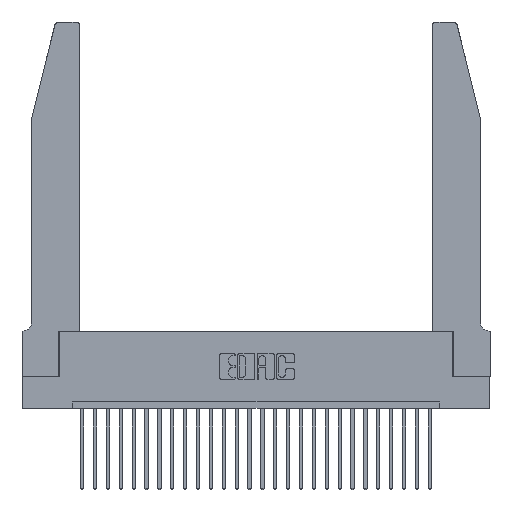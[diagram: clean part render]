
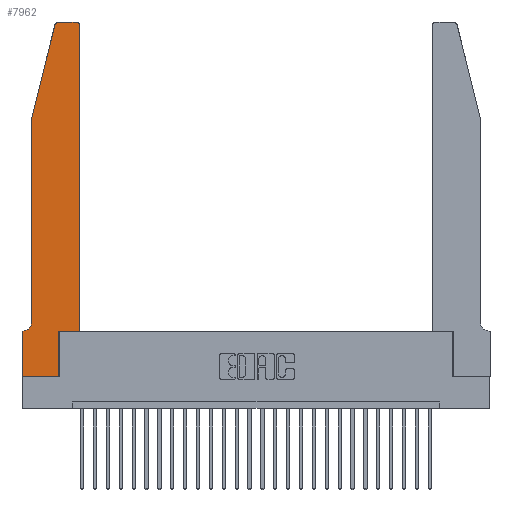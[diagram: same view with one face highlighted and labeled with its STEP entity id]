
A CAD part, top view. The second image highlights one B-rep face of the part: STEP entity #7962.
In plain terms, the highlighted planar face has unit normal (0, 0, 1).
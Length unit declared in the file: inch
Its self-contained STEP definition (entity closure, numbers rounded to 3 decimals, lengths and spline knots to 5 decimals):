
#23 = CARTESIAN_POINT ( 'NONE',  ( 0.0055, 0.42, 0.37 ) ) ;
#168 = CARTESIAN_POINT ( 'NONE',  ( 0.2865, 0.35, 0.37 ) ) ;
#391 = EDGE_CURVE ( 'NONE', #25105, #6199, #17100, .T. ) ;
#398 = FACE_OUTER_BOUND ( 'NONE', #26909, .T. ) ;
#477 = VERTEX_POINT ( 'NONE', #11469 ) ;
#653 = CARTESIAN_POINT ( 'NONE',  ( 0.4205, 2.72, 0.37 ) ) ;
#956 = CIRCLE ( 'NONE', #12991, 0.03 ) ;
#1364 = EDGE_CURVE ( 'NONE', #17092, #24088, #25146, .T. ) ;
#1697 = VECTOR ( 'NONE', #10542, 39.37008 ) ;
#2000 = ORIENTED_EDGE ( 'NONE', *, *, #7348, .T. ) ;
#2100 = EDGE_CURVE ( 'NONE', #6119, #6591, #956, .T. ) ;
#2152 = VERTEX_POINT ( 'NONE', #21927 ) ;
#2568 = DIRECTION ( 'NONE',  ( 0., 0., 1. ) ) ;
#2609 = VECTOR ( 'NONE', #7868, 39.37008 ) ;
#2781 = CARTESIAN_POINT ( 'NONE',  ( 0.0055, 0.35, 0.37 ) ) ;
#4264 = AXIS2_PLACEMENT_3D ( 'NONE', #653, #2568, #6872 ) ;
#4354 = CARTESIAN_POINT ( 'NONE',  ( 0.25487, 2.72718, 0.37 ) ) ;
#4357 = DIRECTION ( 'NONE',  ( 0., 0., -1. ) ) ;
#5154 = DIRECTION ( 'NONE',  ( 0., 0., 1. ) ) ;
#5604 = EDGE_CURVE ( 'NONE', #6199, #19253, #10950, .T. ) ;
#5846 = ORIENTED_EDGE ( 'NONE', *, *, #10791, .T. ) ;
#5909 = VECTOR ( 'NONE', #23273, 39.37008 ) ;
#6119 = VERTEX_POINT ( 'NONE', #7009 ) ;
#6199 = VERTEX_POINT ( 'NONE', #15325 ) ;
#6318 = CARTESIAN_POINT ( 'NONE',  ( 0.0755, 0.35, 0.37 ) ) ;
#6411 = ORIENTED_EDGE ( 'NONE', *, *, #20065, .T. ) ;
#6591 = VERTEX_POINT ( 'NONE', #4354 ) ;
#6872 = DIRECTION ( 'NONE',  ( 1., 0., 0. ) ) ;
#6919 = EDGE_CURVE ( 'NONE', #12487, #25379, #16884, .T. ) ;
#6983 = DIRECTION ( 'NONE',  ( 1., 0., 0. ) ) ;
#7009 = CARTESIAN_POINT ( 'NONE',  ( 0.284, 2.75, 0.37 ) ) ;
#7058 = CARTESIAN_POINT ( 'NONE',  ( 0.284, 2.72, 0.37 ) ) ;
#7182 = DIRECTION ( 'NONE',  ( 1., 0., 0. ) ) ;
#7336 = CARTESIAN_POINT ( 'NONE',  ( 0.0755, 0.42, 0.37 ) ) ;
#7348 = EDGE_CURVE ( 'NONE', #25379, #17092, #19208, .T. ) ;
#7567 = ORIENTED_EDGE ( 'NONE', *, *, #13191, .T. ) ;
#7577 = ORIENTED_EDGE ( 'NONE', *, *, #1364, .T. ) ;
#7868 = DIRECTION ( 'NONE',  ( -0.239, -0.971, 0. ) ) ;
#7962 = ADVANCED_FACE ( 'NONE', ( #398 ), #11408, .T. ) ;
#8135 = ORIENTED_EDGE ( 'NONE', *, *, #6919, .T. ) ;
#8863 = VECTOR ( 'NONE', #11765, 39.37008 ) ;
#10542 = DIRECTION ( 'NONE',  ( -1., 0., 0. ) ) ;
#10791 = EDGE_CURVE ( 'NONE', #6591, #12487, #27391, .T. ) ;
#10950 = LINE ( 'NONE', #14642, #5909 ) ;
#11408 = PLANE ( 'NONE',  #21002 ) ;
#11469 = CARTESIAN_POINT ( 'NONE',  ( 0.4505, 2.72, 0.37 ) ) ;
#11477 = DIRECTION ( 'NONE',  ( 0., 0., 1. ) ) ;
#11765 = DIRECTION ( 'NONE',  ( 0., -1., 0. ) ) ;
#12487 = VERTEX_POINT ( 'NONE', #23101 ) ;
#12876 = EDGE_CURVE ( 'NONE', #2152, #25105, #24219, .T. ) ;
#12991 = AXIS2_PLACEMENT_3D ( 'NONE', #7058, #11477, #6983 ) ;
#13191 = EDGE_CURVE ( 'NONE', #24088, #2152, #14501, .T. ) ;
#13515 = CARTESIAN_POINT ( 'NONE',  ( 0., 0.35, 0.37 ) ) ;
#13733 = VERTEX_POINT ( 'NONE', #18047 ) ;
#14284 = LINE ( 'NONE', #16017, #19633 ) ;
#14501 = LINE ( 'NONE', #22498, #8863 ) ;
#14642 = CARTESIAN_POINT ( 'NONE',  ( 0.4505, 0.35, 0.37 ) ) ;
#14864 = CARTESIAN_POINT ( 'NONE',  ( 0.4505, 0.35, 0.37 ) ) ;
#15325 = CARTESIAN_POINT ( 'NONE',  ( 0.2865, 0.35, 0.37 ) ) ;
#16017 = CARTESIAN_POINT ( 'NONE',  ( 0.2605, 2.75, 0.37 ) ) ;
#16089 = VECTOR ( 'NONE', #17379, 39.37008 ) ;
#16633 = ORIENTED_EDGE ( 'NONE', *, *, #391, .T. ) ;
#16884 = LINE ( 'NONE', #19360, #21246 ) ;
#16989 = CARTESIAN_POINT ( 'NONE',  ( 0.2865, 0., 0.37 ) ) ;
#17092 = VERTEX_POINT ( 'NONE', #2781 ) ;
#17100 = LINE ( 'NONE', #168, #16089 ) ;
#17309 = ORIENTED_EDGE ( 'NONE', *, *, #12876, .T. ) ;
#17379 = DIRECTION ( 'NONE',  ( 0., 1., 0. ) ) ;
#17817 = DIRECTION ( 'NONE',  ( 1., 0., 0. ) ) ;
#17866 = DIRECTION ( 'NONE',  ( 0., -1., 0. ) ) ;
#18047 = CARTESIAN_POINT ( 'NONE',  ( 0.4205, 2.75, 0.37 ) ) ;
#18117 = ORIENTED_EDGE ( 'NONE', *, *, #5604, .T. ) ;
#18612 = LINE ( 'NONE', #27378, #24619 ) ;
#18694 = CARTESIAN_POINT ( 'NONE',  ( 0.0755, 2., 0.37 ) ) ;
#19208 = CIRCLE ( 'NONE', #27432, 0.07 ) ;
#19253 = VERTEX_POINT ( 'NONE', #14864 ) ;
#19360 = CARTESIAN_POINT ( 'NONE',  ( 0.0755, 2., 0.37 ) ) ;
#19633 = VECTOR ( 'NONE', #20114, 39.37008 ) ;
#19650 = ORIENTED_EDGE ( 'NONE', *, *, #24928, .T. ) ;
#20065 = EDGE_CURVE ( 'NONE', #13733, #6119, #14284, .T. ) ;
#20114 = DIRECTION ( 'NONE',  ( -1., 0., 0. ) ) ;
#20362 = CARTESIAN_POINT ( 'NONE',  ( 0., 0., 0.37 ) ) ;
#21002 = AXIS2_PLACEMENT_3D ( 'NONE', #13515, #5154, #17817 ) ;
#21246 = VECTOR ( 'NONE', #17866, 39.37008 ) ;
#21710 = CARTESIAN_POINT ( 'NONE',  ( 0., 0.35, 0.37 ) ) ;
#21927 = CARTESIAN_POINT ( 'NONE',  ( 0., 0., 0.37 ) ) ;
#22498 = CARTESIAN_POINT ( 'NONE',  ( 0., 0., 0.37 ) ) ;
#22878 = ORIENTED_EDGE ( 'NONE', *, *, #2100, .T. ) ;
#23101 = CARTESIAN_POINT ( 'NONE',  ( 0.0755, 2., 0.37 ) ) ;
#23156 = DIRECTION ( 'NONE',  ( 0., 1., 0. ) ) ;
#23273 = DIRECTION ( 'NONE',  ( 1., 0., 0. ) ) ;
#23729 = ORIENTED_EDGE ( 'NONE', *, *, #25698, .T. ) ;
#23906 = VECTOR ( 'NONE', #7182, 39.37008 ) ;
#24088 = VERTEX_POINT ( 'NONE', #21710 ) ;
#24219 = LINE ( 'NONE', #20362, #23906 ) ;
#24588 = CIRCLE ( 'NONE', #4264, 0.03 ) ;
#24619 = VECTOR ( 'NONE', #23156, 39.37008 ) ;
#24928 = EDGE_CURVE ( 'NONE', #19253, #477, #18612, .T. ) ;
#25105 = VERTEX_POINT ( 'NONE', #16989 ) ;
#25146 = LINE ( 'NONE', #6318, #1697 ) ;
#25379 = VERTEX_POINT ( 'NONE', #7336 ) ;
#25698 = EDGE_CURVE ( 'NONE', #477, #13733, #24588, .T. ) ;
#26909 = EDGE_LOOP ( 'NONE', ( #6411, #22878, #5846, #8135, #2000, #7577, #7567, #17309, #16633, #18117, #19650, #23729 ) ) ;
#27378 = CARTESIAN_POINT ( 'NONE',  ( 0.4505, 0.35, 0.37 ) ) ;
#27391 = LINE ( 'NONE', #18694, #2609 ) ;
#27432 = AXIS2_PLACEMENT_3D ( 'NONE', #23, #4357, #27442 ) ;
#27442 = DIRECTION ( 'NONE',  ( -1., 0., 0. ) ) ;
